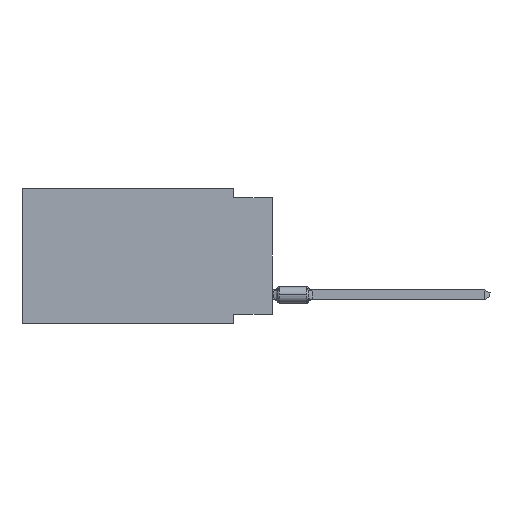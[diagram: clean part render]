
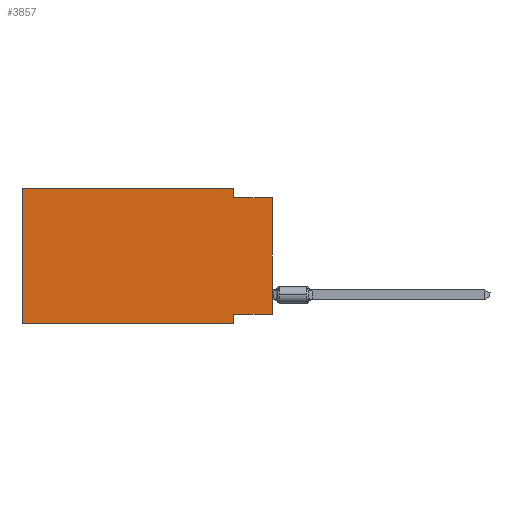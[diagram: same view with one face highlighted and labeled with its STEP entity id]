
A CAD part, left-side view. The second image highlights one B-rep face of the part: STEP entity #3857.
In plain terms, the highlighted planar face has unit normal (-1, 0, 0).
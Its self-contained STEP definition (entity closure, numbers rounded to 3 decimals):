
#101 = CARTESIAN_POINT ( 'NONE',  ( 0., 16.383, -8.89 ) ) ;
#2573 = VECTOR ( 'NONE', #46136, 1000. ) ;
#3748 = DIRECTION ( 'NONE',  ( 0., 0., 1. ) ) ;
#3857 = ADVANCED_FACE ( 'NONE', ( #34183 ), #20043, .F. ) ;
#4751 = DIRECTION ( 'NONE',  ( 0., -1., 0. ) ) ;
#5585 = VERTEX_POINT ( 'NONE', #29090 ) ;
#5674 = LINE ( 'NONE', #15929, #9154 ) ;
#5976 = ORIENTED_EDGE ( 'NONE', *, *, #43963, .T. ) ;
#7407 = LINE ( 'NONE', #11552, #22437 ) ;
#9037 = VERTEX_POINT ( 'NONE', #9259 ) ;
#9154 = VECTOR ( 'NONE', #16643, 1000. ) ;
#9163 = EDGE_CURVE ( 'NONE', #46284, #43431, #36252, .T. ) ;
#9259 = CARTESIAN_POINT ( 'NONE',  ( 0., 2.54, 0. ) ) ;
#10012 = CARTESIAN_POINT ( 'NONE',  ( 0., 2.54, 0. ) ) ;
#10022 = LINE ( 'NONE', #24650, #46960 ) ;
#10052 = EDGE_CURVE ( 'NONE', #9037, #46284, #35836, .T. ) ;
#11552 = CARTESIAN_POINT ( 'NONE',  ( 0., 0., 0. ) ) ;
#11792 = LINE ( 'NONE', #101, #44105 ) ;
#12265 = CARTESIAN_POINT ( 'NONE',  ( 0., 16.383, 0. ) ) ;
#14059 = VECTOR ( 'NONE', #47218, 1000. ) ;
#14090 = VECTOR ( 'NONE', #20747, 1000. ) ;
#14217 = ORIENTED_EDGE ( 'NONE', *, *, #26322, .F. ) ;
#15621 = ORIENTED_EDGE ( 'NONE', *, *, #10052, .F. ) ;
#15929 = CARTESIAN_POINT ( 'NONE',  ( 0., 2.54, -8.89 ) ) ;
#16643 = DIRECTION ( 'NONE',  ( 0., 0., -1. ) ) ;
#16679 = EDGE_LOOP ( 'NONE', ( #5976, #34025, #15621, #43716, #14217, #20113, #27479, #43530 ) ) ;
#18022 = CARTESIAN_POINT ( 'NONE',  ( 0., 0., -0.635 ) ) ;
#18356 = VERTEX_POINT ( 'NONE', #45775 ) ;
#19079 = DIRECTION ( 'NONE',  ( 0., 0., -1. ) ) ;
#20043 = PLANE ( 'NONE',  #37114 ) ;
#20113 = ORIENTED_EDGE ( 'NONE', *, *, #21437, .T. ) ;
#20747 = DIRECTION ( 'NONE',  ( 0., 0., -1. ) ) ;
#21437 = EDGE_CURVE ( 'NONE', #18356, #5585, #11792, .T. ) ;
#22437 = VECTOR ( 'NONE', #3748, 1000. ) ;
#23407 = VERTEX_POINT ( 'NONE', #39249 ) ;
#24650 = CARTESIAN_POINT ( 'NONE',  ( 0., 0., -8.255 ) ) ;
#26169 = EDGE_CURVE ( 'NONE', #47010, #9037, #42245, .T. ) ;
#26322 = EDGE_CURVE ( 'NONE', #18356, #47010, #31519, .T. ) ;
#27479 = ORIENTED_EDGE ( 'NONE', *, *, #41574, .F. ) ;
#27549 = VERTEX_POINT ( 'NONE', #42832 ) ;
#27582 = DIRECTION ( 'NONE',  ( 0., 1., 0. ) ) ;
#29090 = CARTESIAN_POINT ( 'NONE',  ( 0., 2.54, -8.89 ) ) ;
#31519 = LINE ( 'NONE', #46851, #2573 ) ;
#32868 = CARTESIAN_POINT ( 'NONE',  ( 0., 16.383, 0. ) ) ;
#33944 = DIRECTION ( 'NONE',  ( 0., -1., 0. ) ) ;
#33959 = CARTESIAN_POINT ( 'NONE',  ( 0., 2.54, -0.635 ) ) ;
#34025 = ORIENTED_EDGE ( 'NONE', *, *, #9163, .F. ) ;
#34183 = FACE_OUTER_BOUND ( 'NONE', #16679, .T. ) ;
#35394 = EDGE_CURVE ( 'NONE', #27549, #23407, #10022, .T. ) ;
#35836 = LINE ( 'NONE', #10012, #14090 ) ;
#36252 = LINE ( 'NONE', #43813, #14059 ) ;
#37114 = AXIS2_PLACEMENT_3D ( 'NONE', #12265, #42441, #19079 ) ;
#39249 = CARTESIAN_POINT ( 'NONE',  ( 0., 2.54, -8.255 ) ) ;
#40717 = VECTOR ( 'NONE', #4751, 1000. ) ;
#41574 = EDGE_CURVE ( 'NONE', #23407, #5585, #5674, .T. ) ;
#42245 = LINE ( 'NONE', #44939, #40717 ) ;
#42441 = DIRECTION ( 'NONE',  ( 1., 0., 0. ) ) ;
#42832 = CARTESIAN_POINT ( 'NONE',  ( 0., 0., -8.255 ) ) ;
#43431 = VERTEX_POINT ( 'NONE', #18022 ) ;
#43530 = ORIENTED_EDGE ( 'NONE', *, *, #35394, .F. ) ;
#43716 = ORIENTED_EDGE ( 'NONE', *, *, #26169, .F. ) ;
#43813 = CARTESIAN_POINT ( 'NONE',  ( 0., 0., -0.635 ) ) ;
#43963 = EDGE_CURVE ( 'NONE', #27549, #43431, #7407, .T. ) ;
#44105 = VECTOR ( 'NONE', #33944, 1000. ) ;
#44939 = CARTESIAN_POINT ( 'NONE',  ( 0., 16.383, 0. ) ) ;
#45775 = CARTESIAN_POINT ( 'NONE',  ( 0., 16.383, -8.89 ) ) ;
#46136 = DIRECTION ( 'NONE',  ( 0., 0., 1. ) ) ;
#46284 = VERTEX_POINT ( 'NONE', #33959 ) ;
#46851 = CARTESIAN_POINT ( 'NONE',  ( 0., 16.383, 0. ) ) ;
#46960 = VECTOR ( 'NONE', #27582, 1000. ) ;
#47010 = VERTEX_POINT ( 'NONE', #32868 ) ;
#47218 = DIRECTION ( 'NONE',  ( 0., -1., 0. ) ) ;
